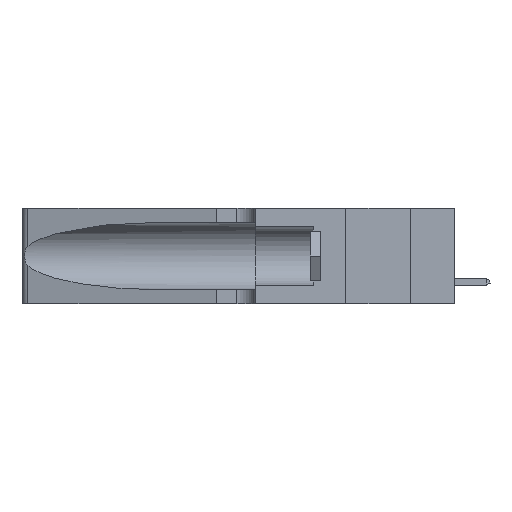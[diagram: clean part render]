
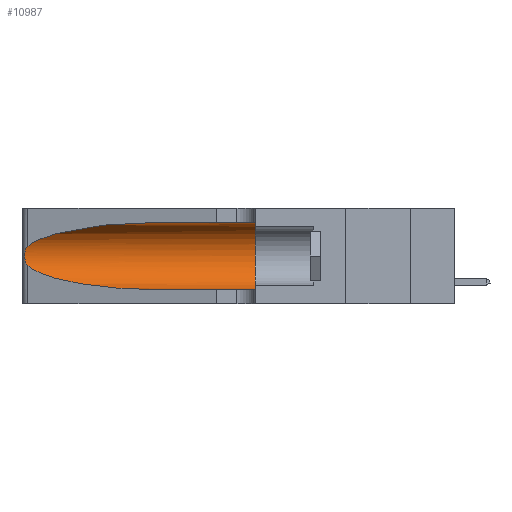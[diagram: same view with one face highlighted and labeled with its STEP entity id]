
A CAD part, left-side view. The second image highlights one B-rep face of the part: STEP entity #10987.
In plain terms, the highlighted cylindrical face has radius 3.308 mm (diameter 6.617 mm), a partial arc.
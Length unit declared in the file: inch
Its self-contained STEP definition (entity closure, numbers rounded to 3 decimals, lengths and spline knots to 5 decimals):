
#16 = CARTESIAN_POINT ( 'NONE',  ( 0.2373, 1.15595, 0.28018 ) ) ;
#109 = VECTOR ( 'NONE', #15245, 39.37008 ) ;
#577 = EDGE_CURVE ( 'NONE', #17605, #1002, #11928, .T. ) ;
#1002 = VERTEX_POINT ( 'NONE', #19229 ) ;
#1232 =( BOUNDED_CURVE ( )  B_SPLINE_CURVE ( 3, ( #8476, #22537, #16, #21099 ),
 .UNSPECIFIED., .F., .F. ) 
 B_SPLINE_CURVE_WITH_KNOTS ( ( 4, 4 ),
 ( 1.5708, 2.84003 ),
 .UNSPECIFIED. ) 
 CURVE ( )  GEOMETRIC_REPRESENTATION_ITEM ( )  RATIONAL_B_SPLINE_CURVE ( ( 1., 0.87, 0.87, 1. ) ) 
 REPRESENTATION_ITEM ( '' )  );
#2709 = CARTESIAN_POINT ( 'NONE',  ( 0.1305, 1.61858, 0.185 ) ) ;
#2719 = CARTESIAN_POINT ( 'NONE',  ( 0.25787, 1.23484, 0.2124 ) ) ;
#3055 = ORIENTED_EDGE ( 'NONE', *, *, #6072, .T. ) ;
#3361 = EDGE_CURVE ( 'NONE', #7515, #6193, #13480, .T. ) ;
#3394 = DIRECTION ( 'NONE',  ( 0., 0., -1. ) ) ;
#4170 = CARTESIAN_POINT ( 'NONE',  ( 0.25639, 1.23184, 0.21858 ) ) ;
#4382 = ORIENTED_EDGE ( 'NONE', *, *, #18554, .F. ) ;
#4932 = CARTESIAN_POINT ( 'NONE',  ( 0.25487, 1.22718, 0.22369 ) ) ;
#5015 = VERTEX_POINT ( 'NONE', #4932 ) ;
#5659 = CARTESIAN_POINT ( 'NONE',  ( 0.1305, 0.35, 0.05475 ) ) ;
#5867 = EDGE_CURVE ( 'NONE', #5015, #7515, #9394, .T. ) ;
#6072 = EDGE_CURVE ( 'NONE', #6193, #18297, #8303, .T. ) ;
#6193 = VERTEX_POINT ( 'NONE', #21705 ) ;
#7515 = VERTEX_POINT ( 'NONE', #12374 ) ;
#7570 = CARTESIAN_POINT ( 'NONE',  ( 0.1305, 0.35, 0.185 ) ) ;
#7932 = CARTESIAN_POINT ( 'NONE',  ( 0.1305, 1.61858, 0.31525 ) ) ;
#7999 = CARTESIAN_POINT ( 'NONE',  ( 0.25854, 1.2359, 0.20912 ) ) ;
#8232 = AXIS2_PLACEMENT_3D ( 'NONE', #2709, #22067, #3394 ) ;
#8303 = LINE ( 'NONE', #14080, #19349 ) ;
#8476 = CARTESIAN_POINT ( 'NONE',  ( 0.1305, 0.72297, 0.31525 ) ) ;
#9072 = EDGE_CURVE ( 'NONE', #17605, #5015, #1232, .T. ) ;
#9394 = B_SPLINE_CURVE_WITH_KNOTS ( 'NONE', 3,
 ( #12999, #13223, #4170, #2719, #7999, #18341, #21857, #20103, #14995, #11224, #16790, #20331, #21775, #9773 ),
 .UNSPECIFIED., .F., .F.,
 ( 4, 2, 2, 2, 2, 2, 4 ),
 ( 0., 0.00027, 0.00053, 0.00107, 0.0016, 0.00187, 0.00214 ),
 .UNSPECIFIED. ) ;
#9488 = DIRECTION ( 'NONE',  ( 0., 1., 0. ) ) ;
#9727 = ORIENTED_EDGE ( 'NONE', *, *, #3361, .T. ) ;
#9773 = CARTESIAN_POINT ( 'NONE',  ( 0.25487, 1.22718, 0.14631 ) ) ;
#10987 = ADVANCED_FACE ( 'NONE', ( #21975 ), #19557, .F. ) ;
#11089 = DIRECTION ( 'NONE',  ( 0., 0., 1. ) ) ;
#11224 = CARTESIAN_POINT ( 'NONE',  ( 0.25856, 1.23593, 0.16098 ) ) ;
#11825 = CARTESIAN_POINT ( 'NONE',  ( 0.18966, 0.96281, 0.05475 ) ) ;
#11928 = LINE ( 'NONE', #7932, #109 ) ;
#12374 = CARTESIAN_POINT ( 'NONE',  ( 0.25487, 1.22718, 0.14631 ) ) ;
#12814 = ORIENTED_EDGE ( 'NONE', *, *, #577, .F. ) ;
#12999 = CARTESIAN_POINT ( 'NONE',  ( 0.25487, 1.22718, 0.22369 ) ) ;
#13223 = CARTESIAN_POINT ( 'NONE',  ( 0.25555, 1.22994, 0.2215 ) ) ;
#13480 =( BOUNDED_CURVE ( )  B_SPLINE_CURVE ( 3, ( #18874, #18954, #11825, #13600 ),
 .UNSPECIFIED., .F., .T. ) 
 B_SPLINE_CURVE_WITH_KNOTS ( ( 4, 4 ),
 ( 3.44316, 4.71239 ),
 .UNSPECIFIED. ) 
 CURVE ( )  GEOMETRIC_REPRESENTATION_ITEM ( )  RATIONAL_B_SPLINE_CURVE ( ( 1., 0.87, 0.87, 1. ) ) 
 REPRESENTATION_ITEM ( '' )  );
#13600 = CARTESIAN_POINT ( 'NONE',  ( 0.1305, 0.72297, 0.05475 ) ) ;
#13806 = ORIENTED_EDGE ( 'NONE', *, *, #5867, .T. ) ;
#14080 = CARTESIAN_POINT ( 'NONE',  ( 0.1305, 1.61858, 0.05475 ) ) ;
#14958 = EDGE_LOOP ( 'NONE', ( #16328, #13806, #9727, #3055, #4382, #12814 ) ) ;
#14995 = CARTESIAN_POINT ( 'NONE',  ( 0.26017, 1.23833, 0.17102 ) ) ;
#15245 = DIRECTION ( 'NONE',  ( 0., -1., 0. ) ) ;
#15790 = DIRECTION ( 'NONE',  ( 0., -1., 0. ) ) ;
#16328 = ORIENTED_EDGE ( 'NONE', *, *, #9072, .T. ) ;
#16397 = CARTESIAN_POINT ( 'NONE',  ( 0.1305, 0.72297, 0.31525 ) ) ;
#16790 = CARTESIAN_POINT ( 'NONE',  ( 0.25789, 1.23486, 0.15765 ) ) ;
#17605 = VERTEX_POINT ( 'NONE', #16397 ) ;
#18297 = VERTEX_POINT ( 'NONE', #5659 ) ;
#18341 = CARTESIAN_POINT ( 'NONE',  ( 0.26018, 1.23835, 0.19895 ) ) ;
#18554 = EDGE_CURVE ( 'NONE', #1002, #18297, #20367, .T. ) ;
#18874 = CARTESIAN_POINT ( 'NONE',  ( 0.25487, 1.22718, 0.14631 ) ) ;
#18954 = CARTESIAN_POINT ( 'NONE',  ( 0.2373, 1.15595, 0.08982 ) ) ;
#19229 = CARTESIAN_POINT ( 'NONE',  ( 0.1305, 0.35, 0.31525 ) ) ;
#19349 = VECTOR ( 'NONE', #15790, 39.37008 ) ;
#19557 = CYLINDRICAL_SURFACE ( 'NONE', #8232, 0.13025 ) ;
#20103 = CARTESIAN_POINT ( 'NONE',  ( 0.26075, 1.23896, 0.178 ) ) ;
#20331 = CARTESIAN_POINT ( 'NONE',  ( 0.25639, 1.23186, 0.15144 ) ) ;
#20367 = CIRCLE ( 'NONE', #20566, 0.13025 ) ;
#20566 = AXIS2_PLACEMENT_3D ( 'NONE', #7570, #9488, #11089 ) ;
#21099 = CARTESIAN_POINT ( 'NONE',  ( 0.25487, 1.22718, 0.22369 ) ) ;
#21705 = CARTESIAN_POINT ( 'NONE',  ( 0.1305, 0.72297, 0.05475 ) ) ;
#21775 = CARTESIAN_POINT ( 'NONE',  ( 0.25555, 1.22993, 0.14849 ) ) ;
#21857 = CARTESIAN_POINT ( 'NONE',  ( 0.26075, 1.23896, 0.19203 ) ) ;
#21975 = FACE_OUTER_BOUND ( 'NONE', #14958, .T. ) ;
#22067 = DIRECTION ( 'NONE',  ( 0., -1., 0. ) ) ;
#22537 = CARTESIAN_POINT ( 'NONE',  ( 0.18966, 0.96281, 0.31525 ) ) ;
